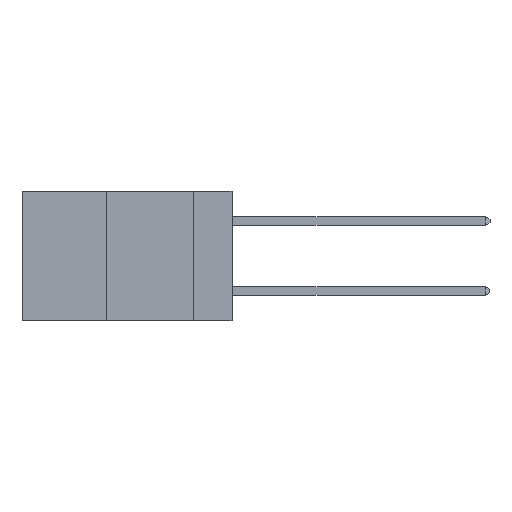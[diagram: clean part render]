
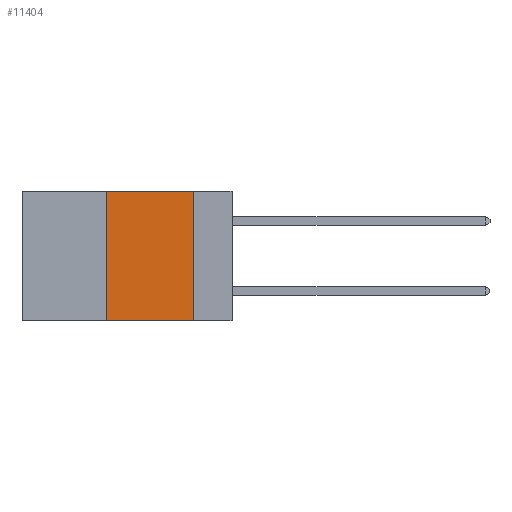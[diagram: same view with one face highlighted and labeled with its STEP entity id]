
A CAD part, left-side view. The second image highlights one B-rep face of the part: STEP entity #11404.
In plain terms, the highlighted planar face has unit normal (-1, 0, 0).
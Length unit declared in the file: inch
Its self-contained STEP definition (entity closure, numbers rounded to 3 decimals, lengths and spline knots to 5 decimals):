
#246 = DIRECTION ( 'NONE',  ( 1., 0., 0. ) ) ;
#360 = CARTESIAN_POINT ( 'NONE',  ( 0., 0.11, 0. ) ) ;
#915 = DIRECTION ( 'NONE',  ( 0., 0., 1. ) ) ;
#992 = CARTESIAN_POINT ( 'NONE',  ( 0., 0.36, 0. ) ) ;
#1850 = EDGE_CURVE ( 'NONE', #9255, #8160, #13507, .T. ) ;
#2304 = ORIENTED_EDGE ( 'NONE', *, *, #2567, .T. ) ;
#2567 = EDGE_CURVE ( 'NONE', #9255, #6347, #6663, .T. ) ;
#2720 = CARTESIAN_POINT ( 'NONE',  ( 0., 0.6, -0.37 ) ) ;
#2738 = DIRECTION ( 'NONE',  ( 0., -1., 0. ) ) ;
#3127 = DIRECTION ( 'NONE',  ( 0., -1., 0. ) ) ;
#3250 = CARTESIAN_POINT ( 'NONE',  ( 0., 0.36, -0.37 ) ) ;
#4539 = CARTESIAN_POINT ( 'NONE',  ( 0., 0.36, 0. ) ) ;
#4629 = PLANE ( 'NONE',  #4931 ) ;
#4723 = VERTEX_POINT ( 'NONE', #360 ) ;
#4876 = ORIENTED_EDGE ( 'NONE', *, *, #9241, .F. ) ;
#4931 = AXIS2_PLACEMENT_3D ( 'NONE', #6726, #246, #7804 ) ;
#6157 = EDGE_LOOP ( 'NONE', ( #4876, #8483, #9143, #2304 ) ) ;
#6330 = CARTESIAN_POINT ( 'NONE',  ( 0., 0.11, -0.37 ) ) ;
#6347 = VERTEX_POINT ( 'NONE', #6330 ) ;
#6432 = CARTESIAN_POINT ( 'NONE',  ( 0., 0.11, 0. ) ) ;
#6663 = LINE ( 'NONE', #2720, #12152 ) ;
#6726 = CARTESIAN_POINT ( 'NONE',  ( 0., 0.6, 0. ) ) ;
#7387 = CARTESIAN_POINT ( 'NONE',  ( 0., 0.6, 0. ) ) ;
#7804 = DIRECTION ( 'NONE',  ( 0., 0., -1. ) ) ;
#8160 = VERTEX_POINT ( 'NONE', #4539 ) ;
#8457 = VECTOR ( 'NONE', #9571, 39.37008 ) ;
#8483 = ORIENTED_EDGE ( 'NONE', *, *, #9146, .F. ) ;
#9143 = ORIENTED_EDGE ( 'NONE', *, *, #1850, .F. ) ;
#9146 = EDGE_CURVE ( 'NONE', #8160, #4723, #12461, .T. ) ;
#9241 = EDGE_CURVE ( 'NONE', #4723, #6347, #11193, .T. ) ;
#9255 = VERTEX_POINT ( 'NONE', #3250 ) ;
#9571 = DIRECTION ( 'NONE',  ( 0., 0., -1. ) ) ;
#9708 = VECTOR ( 'NONE', #3127, 39.37008 ) ;
#10881 = VECTOR ( 'NONE', #915, 39.37008 ) ;
#11193 = LINE ( 'NONE', #6432, #8457 ) ;
#11404 = ADVANCED_FACE ( 'NONE', ( #12094 ), #4629, .F. ) ;
#12094 = FACE_OUTER_BOUND ( 'NONE', #6157, .T. ) ;
#12152 = VECTOR ( 'NONE', #2738, 39.37008 ) ;
#12461 = LINE ( 'NONE', #7387, #9708 ) ;
#13507 = LINE ( 'NONE', #992, #10881 ) ;
